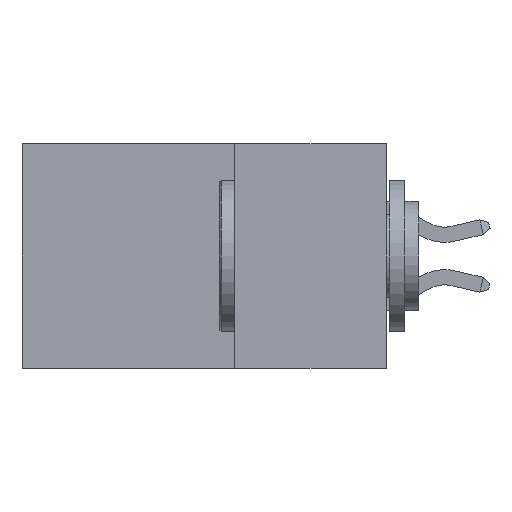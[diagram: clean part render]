
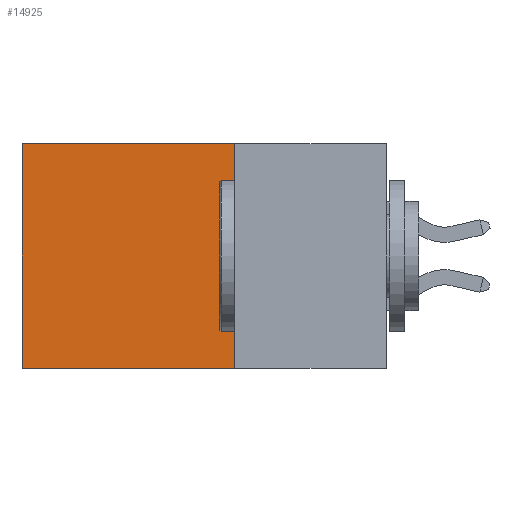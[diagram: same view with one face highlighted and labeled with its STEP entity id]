
A CAD part, left-side view. The second image highlights one B-rep face of the part: STEP entity #14925.
In plain terms, the highlighted planar face has unit normal (-1, 0, 0).
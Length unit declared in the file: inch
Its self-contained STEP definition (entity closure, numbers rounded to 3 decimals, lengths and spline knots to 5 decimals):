
#1088 = VECTOR ( 'NONE', #16697, 39.37008 ) ;
#1884 = CARTESIAN_POINT ( 'NONE',  ( 0.298, 0.25, 0. ) ) ;
#2149 = ORIENTED_EDGE ( 'NONE', *, *, #10032, .F. ) ;
#2153 = VECTOR ( 'NONE', #3539, 39.37008 ) ;
#2471 = CARTESIAN_POINT ( 'NONE',  ( 0.298, 0.25, 0. ) ) ;
#2690 = VECTOR ( 'NONE', #15495, 39.37008 ) ;
#3539 = DIRECTION ( 'NONE',  ( 0., 0., -1. ) ) ;
#3982 = CARTESIAN_POINT ( 'NONE',  ( 0.298, 0.25, 0. ) ) ;
#4137 = DIRECTION ( 'NONE',  ( 0., 0., -1. ) ) ;
#5096 = AXIS2_PLACEMENT_3D ( 'NONE', #2471, #13924, #4137 ) ;
#5353 = EDGE_CURVE ( 'NONE', #5654, #17367, #19028, .T. ) ;
#5497 = LINE ( 'NONE', #7248, #14157 ) ;
#5654 = VERTEX_POINT ( 'NONE', #16674 ) ;
#5909 = VERTEX_POINT ( 'NONE', #3982 ) ;
#6316 = VERTEX_POINT ( 'NONE', #20991 ) ;
#6605 = EDGE_CURVE ( 'NONE', #6316, #17367, #5497, .T. ) ;
#7248 = CARTESIAN_POINT ( 'NONE',  ( 0.298, 0.25, -0.37 ) ) ;
#10032 = EDGE_CURVE ( 'NONE', #5909, #6316, #10833, .T. ) ;
#10084 = EDGE_CURVE ( 'NONE', #5909, #5654, #18510, .T. ) ;
#10205 = DIRECTION ( 'NONE',  ( 0., 1., 0. ) ) ;
#10833 = LINE ( 'NONE', #1884, #2153 ) ;
#11392 = EDGE_LOOP ( 'NONE', ( #18994, #16550, #2149, #21020 ) ) ;
#11755 = CARTESIAN_POINT ( 'NONE',  ( 0.298, 0.25, 0. ) ) ;
#12708 = FACE_OUTER_BOUND ( 'NONE', #11392, .T. ) ;
#13924 = DIRECTION ( 'NONE',  ( 1., 0., 0. ) ) ;
#14157 = VECTOR ( 'NONE', #10205, 39.37008 ) ;
#14925 = ADVANCED_FACE ( 'NONE', ( #12708 ), #20376, .F. ) ;
#15495 = DIRECTION ( 'NONE',  ( 0., 0., -1. ) ) ;
#16550 = ORIENTED_EDGE ( 'NONE', *, *, #6605, .F. ) ;
#16674 = CARTESIAN_POINT ( 'NONE',  ( 0.298, 0.6, 0. ) ) ;
#16697 = DIRECTION ( 'NONE',  ( 0., 1., 0. ) ) ;
#16887 = CARTESIAN_POINT ( 'NONE',  ( 0.298, 0.6, -0.37 ) ) ;
#17367 = VERTEX_POINT ( 'NONE', #16887 ) ;
#18510 = LINE ( 'NONE', #11755, #1088 ) ;
#18994 = ORIENTED_EDGE ( 'NONE', *, *, #5353, .T. ) ;
#19028 = LINE ( 'NONE', #21050, #2690 ) ;
#20376 = PLANE ( 'NONE',  #5096 ) ;
#20991 = CARTESIAN_POINT ( 'NONE',  ( 0.298, 0.25, -0.37 ) ) ;
#21020 = ORIENTED_EDGE ( 'NONE', *, *, #10084, .T. ) ;
#21050 = CARTESIAN_POINT ( 'NONE',  ( 0.298, 0.6, 0. ) ) ;
